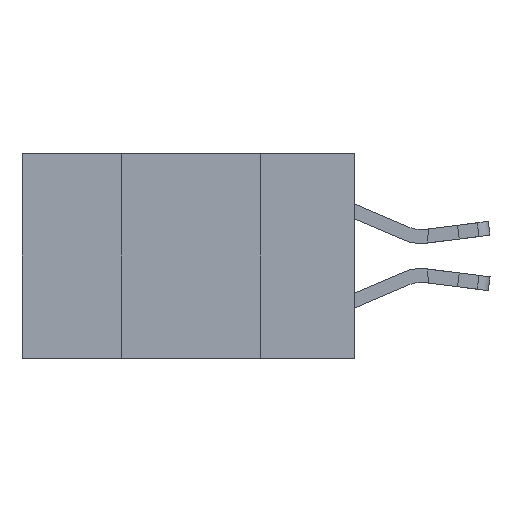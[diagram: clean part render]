
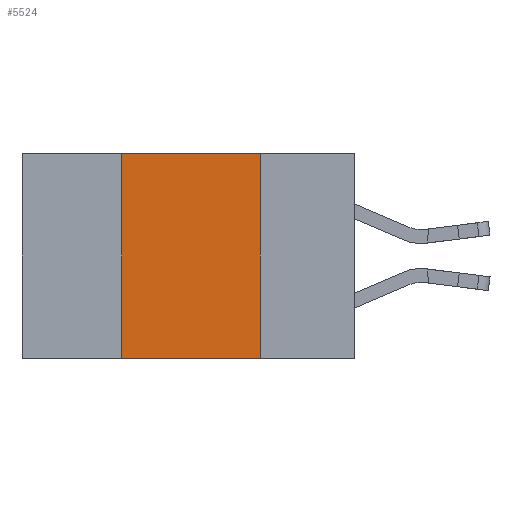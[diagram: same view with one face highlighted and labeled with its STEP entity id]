
A CAD part, left-side view. The second image highlights one B-rep face of the part: STEP entity #5524.
In plain terms, the highlighted planar face has unit normal (-1, 0, 0).
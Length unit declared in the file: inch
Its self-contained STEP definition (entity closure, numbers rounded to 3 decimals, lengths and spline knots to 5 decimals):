
#179 = VECTOR ( 'NONE', #8255, 39.37008 ) ;
#654 = ORIENTED_EDGE ( 'NONE', *, *, #3557, .F. ) ;
#841 = VECTOR ( 'NONE', #5437, 39.37008 ) ;
#1324 = DIRECTION ( 'NONE',  ( 0., 0., -1. ) ) ;
#2009 = EDGE_LOOP ( 'NONE', ( #9860, #654, #15538, #2082 ) ) ;
#2063 = PLANE ( 'NONE',  #4486 ) ;
#2082 = ORIENTED_EDGE ( 'NONE', *, *, #16597, .T. ) ;
#2753 = VERTEX_POINT ( 'NONE', #3178 ) ;
#2772 = CARTESIAN_POINT ( 'NONE',  ( 0., 0.17, 0. ) ) ;
#3178 = CARTESIAN_POINT ( 'NONE',  ( 0., 0.42, 0. ) ) ;
#3557 = EDGE_CURVE ( 'NONE', #2753, #4380, #14930, .T. ) ;
#4359 = EDGE_CURVE ( 'NONE', #4380, #17296, #5949, .T. ) ;
#4380 = VERTEX_POINT ( 'NONE', #2772 ) ;
#4486 = AXIS2_PLACEMENT_3D ( 'NONE', #4900, #6301, #7835 ) ;
#4746 = CARTESIAN_POINT ( 'NONE',  ( 0., 0.42, -0.37 ) ) ;
#4900 = CARTESIAN_POINT ( 'NONE',  ( 0., 0.6, 0. ) ) ;
#5437 = DIRECTION ( 'NONE',  ( 0., 0., 1. ) ) ;
#5524 = ADVANCED_FACE ( 'NONE', ( #10518 ), #2063, .F. ) ;
#5949 = LINE ( 'NONE', #10003, #13822 ) ;
#6301 = DIRECTION ( 'NONE',  ( 1., 0., 0. ) ) ;
#6958 = CARTESIAN_POINT ( 'NONE',  ( 0., 0.42, 0. ) ) ;
#7081 = CARTESIAN_POINT ( 'NONE',  ( 0., 0.6, -0.37 ) ) ;
#7835 = DIRECTION ( 'NONE',  ( 0., 0., -1. ) ) ;
#8255 = DIRECTION ( 'NONE',  ( 0., -1., 0. ) ) ;
#9860 = ORIENTED_EDGE ( 'NONE', *, *, #4359, .F. ) ;
#10003 = CARTESIAN_POINT ( 'NONE',  ( 0., 0.17, 0. ) ) ;
#10518 = FACE_OUTER_BOUND ( 'NONE', #2009, .T. ) ;
#12052 = LINE ( 'NONE', #6958, #841 ) ;
#12474 = CARTESIAN_POINT ( 'NONE',  ( 0., 0.6, 0. ) ) ;
#12762 = VECTOR ( 'NONE', #15254, 39.37008 ) ;
#13822 = VECTOR ( 'NONE', #1324, 39.37008 ) ;
#14855 = LINE ( 'NONE', #7081, #179 ) ;
#14930 = LINE ( 'NONE', #12474, #12762 ) ;
#15030 = VERTEX_POINT ( 'NONE', #4746 ) ;
#15254 = DIRECTION ( 'NONE',  ( 0., -1., 0. ) ) ;
#15538 = ORIENTED_EDGE ( 'NONE', *, *, #16542, .F. ) ;
#16542 = EDGE_CURVE ( 'NONE', #15030, #2753, #12052, .T. ) ;
#16597 = EDGE_CURVE ( 'NONE', #15030, #17296, #14855, .T. ) ;
#17044 = CARTESIAN_POINT ( 'NONE',  ( 0., 0.17, -0.37 ) ) ;
#17296 = VERTEX_POINT ( 'NONE', #17044 ) ;
